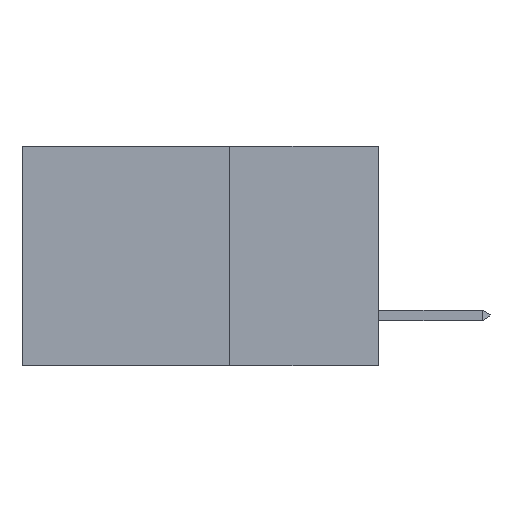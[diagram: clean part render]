
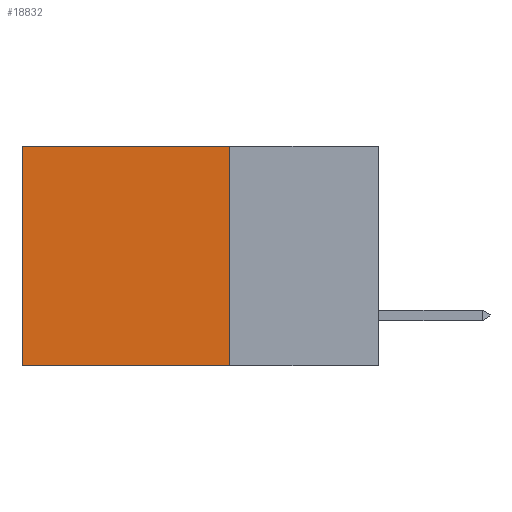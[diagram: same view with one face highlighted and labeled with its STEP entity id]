
A CAD part, left-side view. The second image highlights one B-rep face of the part: STEP entity #18832.
In plain terms, the highlighted planar face has unit normal (-1, 0, 0).
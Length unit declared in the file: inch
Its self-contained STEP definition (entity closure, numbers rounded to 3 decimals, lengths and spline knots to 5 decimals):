
#618 = DIRECTION ( 'NONE',  ( 0., 1., 0. ) ) ;
#781 = ORIENTED_EDGE ( 'NONE', *, *, #3264, .F. ) ;
#1050 = EDGE_CURVE ( 'NONE', #19261, #4444, #9454, .T. ) ;
#1880 = LINE ( 'NONE', #8632, #21316 ) ;
#2494 = VERTEX_POINT ( 'NONE', #10688 ) ;
#2793 = DIRECTION ( 'NONE',  ( 0., 1., 0. ) ) ;
#3264 = EDGE_CURVE ( 'NONE', #4310, #4444, #9916, .T. ) ;
#3766 = LINE ( 'NONE', #11710, #10126 ) ;
#3791 = ORIENTED_EDGE ( 'NONE', *, *, #9703, .T. ) ;
#4310 = VERTEX_POINT ( 'NONE', #17459 ) ;
#4444 = VERTEX_POINT ( 'NONE', #17899 ) ;
#7383 = PLANE ( 'NONE',  #20913 ) ;
#7675 = CARTESIAN_POINT ( 'NONE',  ( 0.298, 0.6, 0. ) ) ;
#7746 = DIRECTION ( 'NONE',  ( 0., 0., -1. ) ) ;
#8632 = CARTESIAN_POINT ( 'NONE',  ( 0.298, 0.25, 0. ) ) ;
#8715 = DIRECTION ( 'NONE',  ( 0., 0., -1. ) ) ;
#9454 = LINE ( 'NONE', #7675, #16833 ) ;
#9703 = EDGE_CURVE ( 'NONE', #2494, #19261, #3766, .T. ) ;
#9916 = LINE ( 'NONE', #14580, #13740 ) ;
#10126 = VECTOR ( 'NONE', #2793, 39.37008 ) ;
#10688 = CARTESIAN_POINT ( 'NONE',  ( 0.298, 0.25, 0. ) ) ;
#10880 = EDGE_CURVE ( 'NONE', #2494, #4310, #1880, .T. ) ;
#10895 = FACE_OUTER_BOUND ( 'NONE', #19234, .T. ) ;
#10991 = DIRECTION ( 'NONE',  ( 1., 0., 0. ) ) ;
#11710 = CARTESIAN_POINT ( 'NONE',  ( 0.298, 0.25, 0. ) ) ;
#13740 = VECTOR ( 'NONE', #618, 39.37008 ) ;
#13897 = ORIENTED_EDGE ( 'NONE', *, *, #10880, .F. ) ;
#14580 = CARTESIAN_POINT ( 'NONE',  ( 0.298, 0.25, -0.37 ) ) ;
#16374 = CARTESIAN_POINT ( 'NONE',  ( 0.298, 0.25, 0. ) ) ;
#16833 = VECTOR ( 'NONE', #7746, 39.37008 ) ;
#17459 = CARTESIAN_POINT ( 'NONE',  ( 0.298, 0.25, -0.37 ) ) ;
#17899 = CARTESIAN_POINT ( 'NONE',  ( 0.298, 0.6, -0.37 ) ) ;
#18832 = ADVANCED_FACE ( 'NONE', ( #10895 ), #7383, .F. ) ;
#19234 = EDGE_LOOP ( 'NONE', ( #21546, #781, #13897, #3791 ) ) ;
#19261 = VERTEX_POINT ( 'NONE', #21410 ) ;
#20913 = AXIS2_PLACEMENT_3D ( 'NONE', #16374, #10991, #21672 ) ;
#21316 = VECTOR ( 'NONE', #8715, 39.37008 ) ;
#21410 = CARTESIAN_POINT ( 'NONE',  ( 0.298, 0.6, 0. ) ) ;
#21546 = ORIENTED_EDGE ( 'NONE', *, *, #1050, .T. ) ;
#21672 = DIRECTION ( 'NONE',  ( 0., 0., -1. ) ) ;
